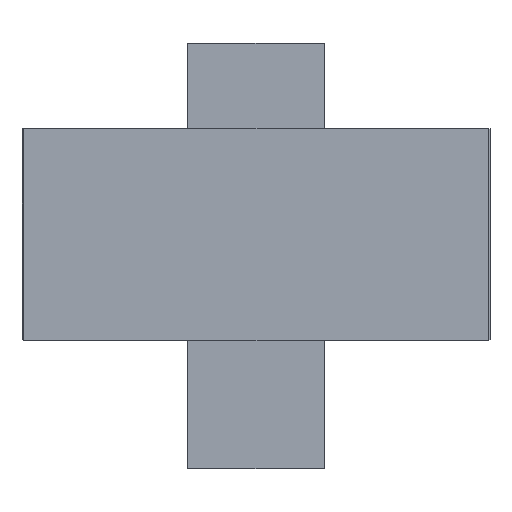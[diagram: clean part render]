
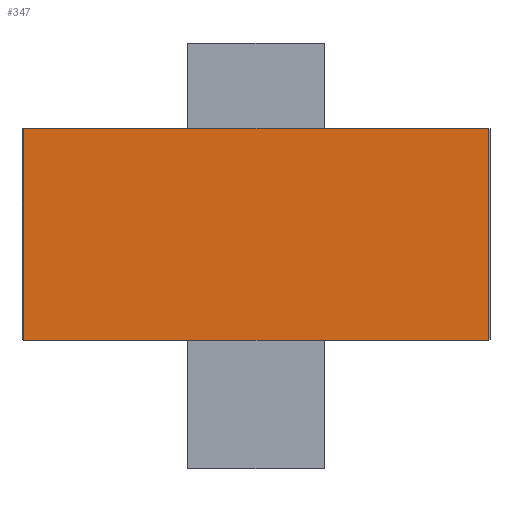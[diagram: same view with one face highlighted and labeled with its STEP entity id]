
A CAD part, front view. The second image highlights one B-rep face of the part: STEP entity #347.
In plain terms, the highlighted planar face has unit normal (0, -1, 0).
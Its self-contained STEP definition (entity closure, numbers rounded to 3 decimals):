
#14 = PLANE ( 'NONE',  #260 ) ;
#18 = VERTEX_POINT ( 'NONE', #623 ) ;
#26 = ORIENTED_EDGE ( 'NONE', *, *, #700, .F. ) ;
#30 = LINE ( 'NONE', #302, #547 ) ;
#106 = VERTEX_POINT ( 'NONE', #627 ) ;
#108 = CARTESIAN_POINT ( 'NONE',  ( -5.918, -1.397, -7.569 ) ) ;
#117 = VECTOR ( 'NONE', #253, 1000. ) ;
#126 = ORIENTED_EDGE ( 'NONE', *, *, #237, .T. ) ;
#172 = DIRECTION ( 'NONE',  ( 0., 0., 1. ) ) ;
#175 = CARTESIAN_POINT ( 'NONE',  ( 5.969, -1.397, -7.569 ) ) ;
#177 = DIRECTION ( 'NONE',  ( 0., 1., 0. ) ) ;
#188 = EDGE_CURVE ( 'NONE', #106, #358, #414, .T. ) ;
#207 = CARTESIAN_POINT ( 'NONE',  ( 5.969, -1.397, -2.159 ) ) ;
#231 = ORIENTED_EDGE ( 'NONE', *, *, #188, .T. ) ;
#237 = EDGE_CURVE ( 'NONE', #687, #106, #436, .T. ) ;
#253 = DIRECTION ( 'NONE',  ( -1., 0., 0. ) ) ;
#260 = AXIS2_PLACEMENT_3D ( 'NONE', #175, #177, #172 ) ;
#296 = DIRECTION ( 'NONE',  ( 0., 0., 1. ) ) ;
#300 = CARTESIAN_POINT ( 'NONE',  ( 5.918, -1.397, -2.159 ) ) ;
#301 = CARTESIAN_POINT ( 'NONE',  ( 5.969, -1.397, -7.569 ) ) ;
#302 = CARTESIAN_POINT ( 'NONE',  ( 5.918, -1.397, -7.569 ) ) ;
#347 = ADVANCED_FACE ( 'NONE', ( #478 ), #14, .F. ) ;
#352 = VECTOR ( 'NONE', #369, 1000. ) ;
#358 = VERTEX_POINT ( 'NONE', #108 ) ;
#369 = DIRECTION ( 'NONE',  ( 0., 0., -1. ) ) ;
#414 = LINE ( 'NONE', #450, #352 ) ;
#436 = LINE ( 'NONE', #207, #780 ) ;
#450 = CARTESIAN_POINT ( 'NONE',  ( -5.918, -1.397, -7.569 ) ) ;
#478 = FACE_OUTER_BOUND ( 'NONE', #716, .T. ) ;
#486 = ORIENTED_EDGE ( 'NONE', *, *, #683, .T. ) ;
#547 = VECTOR ( 'NONE', #296, 1000. ) ;
#623 = CARTESIAN_POINT ( 'NONE',  ( 5.918, -1.397, -7.569 ) ) ;
#627 = CARTESIAN_POINT ( 'NONE',  ( -5.918, -1.397, -2.159 ) ) ;
#683 = EDGE_CURVE ( 'NONE', #18, #687, #30, .T. ) ;
#687 = VERTEX_POINT ( 'NONE', #300 ) ;
#700 = EDGE_CURVE ( 'NONE', #18, #358, #745, .T. ) ;
#702 = DIRECTION ( 'NONE',  ( -1., 0., 0. ) ) ;
#716 = EDGE_LOOP ( 'NONE', ( #126, #231, #26, #486 ) ) ;
#745 = LINE ( 'NONE', #301, #117 ) ;
#780 = VECTOR ( 'NONE', #702, 1000. ) ;
